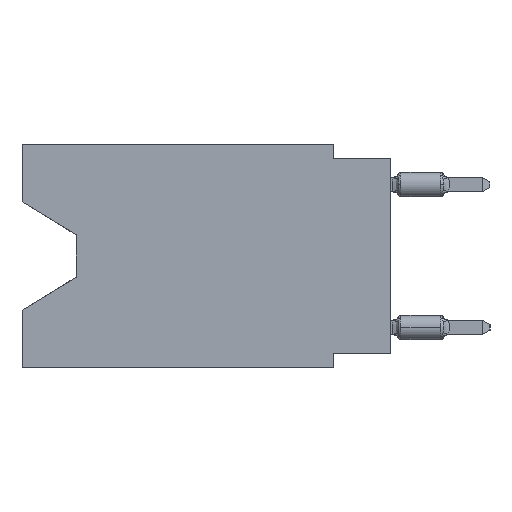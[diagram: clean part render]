
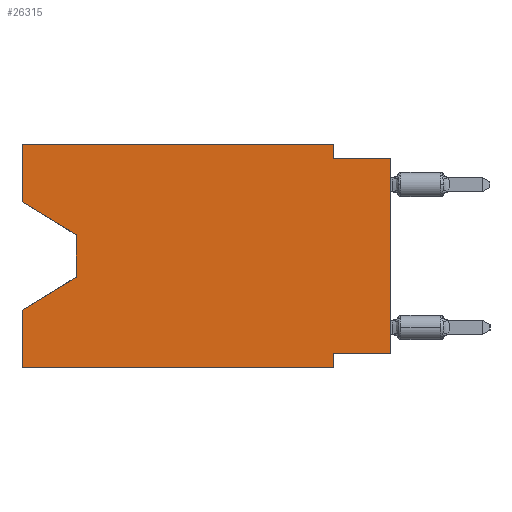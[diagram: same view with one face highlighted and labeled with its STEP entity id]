
A CAD part, left-side view. The second image highlights one B-rep face of the part: STEP entity #26315.
In plain terms, the highlighted planar face has unit normal (-1, 0, 0).
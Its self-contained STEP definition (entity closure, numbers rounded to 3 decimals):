
#391 = CARTESIAN_POINT ( 'NONE',  ( 0., 2.54, 0. ) ) ;
#405 = VERTEX_POINT ( 'NONE', #7065 ) ;
#486 = CARTESIAN_POINT ( 'NONE',  ( 0., 13.97, -4.013 ) ) ;
#650 = LINE ( 'NONE', #35620, #19632 ) ;
#1341 = EDGE_CURVE ( 'NONE', #40345, #17729, #19770, .T. ) ;
#2035 = EDGE_LOOP ( 'NONE', ( #5182, #2202, #21513, #38989, #18526, #31110, #18325, #40269, #31553, #43384, #27736, #8020 ) ) ;
#2202 = ORIENTED_EDGE ( 'NONE', *, *, #1341, .T. ) ;
#2869 = CARTESIAN_POINT ( 'NONE',  ( 0., 2.54, -9.906 ) ) ;
#4099 = FACE_OUTER_BOUND ( 'NONE', #2035, .T. ) ;
#4923 = CARTESIAN_POINT ( 'NONE',  ( 0., 2.54, -9.271 ) ) ;
#5060 = DIRECTION ( 'NONE',  ( 0., 0.855, -0.519 ) ) ;
#5182 = ORIENTED_EDGE ( 'NONE', *, *, #44146, .T. ) ;
#5185 = EDGE_CURVE ( 'NONE', #405, #14578, #43611, .T. ) ;
#5351 = EDGE_CURVE ( 'NONE', #17729, #32430, #13508, .T. ) ;
#6017 = CARTESIAN_POINT ( 'NONE',  ( 0., 16.383, 0. ) ) ;
#6256 = VECTOR ( 'NONE', #26513, 1000. ) ;
#7065 = CARTESIAN_POINT ( 'NONE',  ( 0., 16.383, -2.546 ) ) ;
#8020 = ORIENTED_EDGE ( 'NONE', *, *, #5185, .F. ) ;
#8490 = DIRECTION ( 'NONE',  ( 0., 0., 1. ) ) ;
#9085 = CARTESIAN_POINT ( 'NONE',  ( 0., 13.97, -5.893 ) ) ;
#9532 = CARTESIAN_POINT ( 'NONE',  ( 0., 0., -0.635 ) ) ;
#9763 = VECTOR ( 'NONE', #12226, 1000. ) ;
#9976 = CARTESIAN_POINT ( 'NONE',  ( 0., 16.383, -2.546 ) ) ;
#10173 = VERTEX_POINT ( 'NONE', #4923 ) ;
#11339 = DIRECTION ( 'NONE',  ( 0., 0., -1. ) ) ;
#12226 = DIRECTION ( 'NONE',  ( 0., 0., -1. ) ) ;
#12855 = VECTOR ( 'NONE', #20293, 1000. ) ;
#13218 = VECTOR ( 'NONE', #38979, 1000. ) ;
#13508 = LINE ( 'NONE', #40516, #27090 ) ;
#14578 = VERTEX_POINT ( 'NONE', #6017 ) ;
#15113 = DIRECTION ( 'NONE',  ( 0., -1., 0. ) ) ;
#15600 = CARTESIAN_POINT ( 'NONE',  ( 0., 16.383, 0. ) ) ;
#16163 = PLANE ( 'NONE',  #39170 ) ;
#17151 = EDGE_CURVE ( 'NONE', #21117, #35637, #19931, .T. ) ;
#17729 = VERTEX_POINT ( 'NONE', #9085 ) ;
#17921 = DIRECTION ( 'NONE',  ( 0., -0.855, -0.519 ) ) ;
#18325 = ORIENTED_EDGE ( 'NONE', *, *, #38790, .F. ) ;
#18338 = VERTEX_POINT ( 'NONE', #23957 ) ;
#18526 = ORIENTED_EDGE ( 'NONE', *, *, #47701, .T. ) ;
#19632 = VECTOR ( 'NONE', #39472, 1000. ) ;
#19770 = LINE ( 'NONE', #486, #32977 ) ;
#19931 = LINE ( 'NONE', #391, #9763 ) ;
#20293 = DIRECTION ( 'NONE',  ( 0., 1., 0. ) ) ;
#21117 = VERTEX_POINT ( 'NONE', #46112 ) ;
#21513 = ORIENTED_EDGE ( 'NONE', *, *, #5351, .T. ) ;
#22131 = VERTEX_POINT ( 'NONE', #9532 ) ;
#22315 = VERTEX_POINT ( 'NONE', #40070 ) ;
#22856 = VECTOR ( 'NONE', #17921, 1000. ) ;
#23180 = LINE ( 'NONE', #2869, #23500 ) ;
#23500 = VECTOR ( 'NONE', #11339, 1000. ) ;
#23861 = EDGE_CURVE ( 'NONE', #35637, #22131, #33909, .T. ) ;
#23882 = CARTESIAN_POINT ( 'NONE',  ( 0., 16.383, 0. ) ) ;
#23957 = CARTESIAN_POINT ( 'NONE',  ( 0., 16.383, -9.906 ) ) ;
#26315 = ADVANCED_FACE ( 'NONE', ( #4099 ), #16163, .F. ) ;
#26513 = DIRECTION ( 'NONE',  ( 0., -1., 0. ) ) ;
#26558 = DIRECTION ( 'NONE',  ( 0., 0., 1. ) ) ;
#27090 = VECTOR ( 'NONE', #5060, 1000. ) ;
#27101 = EDGE_CURVE ( 'NONE', #18338, #32430, #30430, .T. ) ;
#27736 = ORIENTED_EDGE ( 'NONE', *, *, #38510, .F. ) ;
#28552 = VECTOR ( 'NONE', #26558, 1000. ) ;
#28793 = LINE ( 'NONE', #35996, #47195 ) ;
#29514 = LINE ( 'NONE', #9976, #22856 ) ;
#30114 = CARTESIAN_POINT ( 'NONE',  ( 0., 16.383, 0. ) ) ;
#30430 = LINE ( 'NONE', #46095, #28552 ) ;
#31110 = ORIENTED_EDGE ( 'NONE', *, *, #41582, .F. ) ;
#31331 = CARTESIAN_POINT ( 'NONE',  ( 0., 13.97, -4.013 ) ) ;
#31553 = ORIENTED_EDGE ( 'NONE', *, *, #23861, .F. ) ;
#32430 = VERTEX_POINT ( 'NONE', #37797 ) ;
#32647 = LINE ( 'NONE', #48809, #12855 ) ;
#32977 = VECTOR ( 'NONE', #35214, 1000. ) ;
#33646 = CARTESIAN_POINT ( 'NONE',  ( 0., 0., -0.635 ) ) ;
#33864 = CARTESIAN_POINT ( 'NONE',  ( 0., 0., -9.271 ) ) ;
#33909 = LINE ( 'NONE', #33646, #41710 ) ;
#35196 = EDGE_CURVE ( 'NONE', #49807, #22131, #28793, .T. ) ;
#35214 = DIRECTION ( 'NONE',  ( 0., 0., -1. ) ) ;
#35620 = CARTESIAN_POINT ( 'NONE',  ( 0., 16.383, -9.906 ) ) ;
#35637 = VERTEX_POINT ( 'NONE', #35673 ) ;
#35673 = CARTESIAN_POINT ( 'NONE',  ( 0., 2.54, -0.635 ) ) ;
#35709 = DIRECTION ( 'NONE',  ( 1., 0., 0. ) ) ;
#35974 = DIRECTION ( 'NONE',  ( 0., 0., -1. ) ) ;
#35996 = CARTESIAN_POINT ( 'NONE',  ( 0., 0., 0. ) ) ;
#37797 = CARTESIAN_POINT ( 'NONE',  ( 0., 16.383, -7.36 ) ) ;
#38510 = EDGE_CURVE ( 'NONE', #14578, #21117, #46044, .T. ) ;
#38790 = EDGE_CURVE ( 'NONE', #49807, #10173, #32647, .T. ) ;
#38979 = DIRECTION ( 'NONE',  ( 0., 0., 1. ) ) ;
#38989 = ORIENTED_EDGE ( 'NONE', *, *, #27101, .F. ) ;
#39170 = AXIS2_PLACEMENT_3D ( 'NONE', #23882, #35709, #35974 ) ;
#39472 = DIRECTION ( 'NONE',  ( 0., -1., 0. ) ) ;
#40070 = CARTESIAN_POINT ( 'NONE',  ( 0., 2.54, -9.906 ) ) ;
#40269 = ORIENTED_EDGE ( 'NONE', *, *, #35196, .T. ) ;
#40345 = VERTEX_POINT ( 'NONE', #31331 ) ;
#40516 = CARTESIAN_POINT ( 'NONE',  ( 0., 13.97, -5.893 ) ) ;
#41582 = EDGE_CURVE ( 'NONE', #10173, #22315, #23180, .T. ) ;
#41710 = VECTOR ( 'NONE', #15113, 1000. ) ;
#43384 = ORIENTED_EDGE ( 'NONE', *, *, #17151, .F. ) ;
#43611 = LINE ( 'NONE', #15600, #13218 ) ;
#44146 = EDGE_CURVE ( 'NONE', #405, #40345, #29514, .T. ) ;
#46044 = LINE ( 'NONE', #30114, #6256 ) ;
#46095 = CARTESIAN_POINT ( 'NONE',  ( 0., 16.383, 0. ) ) ;
#46112 = CARTESIAN_POINT ( 'NONE',  ( 0., 2.54, 0. ) ) ;
#47195 = VECTOR ( 'NONE', #8490, 1000. ) ;
#47701 = EDGE_CURVE ( 'NONE', #18338, #22315, #650, .T. ) ;
#48809 = CARTESIAN_POINT ( 'NONE',  ( 0., 0., -9.271 ) ) ;
#49807 = VERTEX_POINT ( 'NONE', #33864 ) ;
